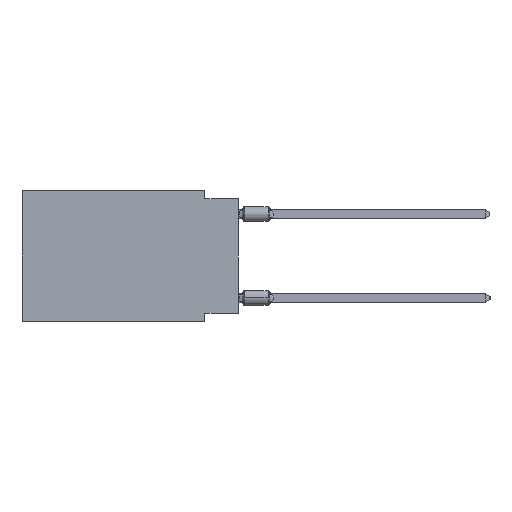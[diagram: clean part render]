
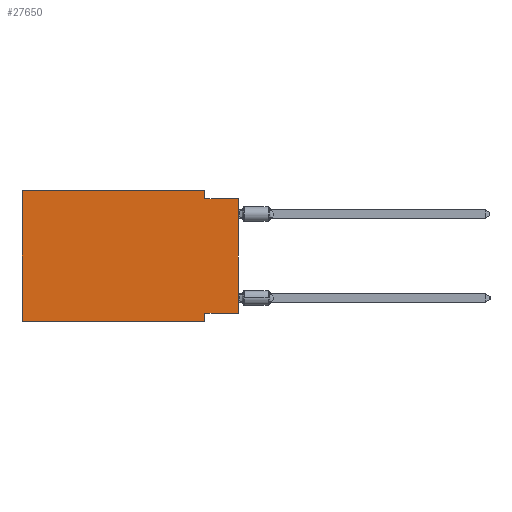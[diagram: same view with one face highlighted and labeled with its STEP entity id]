
A CAD part, left-side view. The second image highlights one B-rep face of the part: STEP entity #27650.
In plain terms, the highlighted planar face has unit normal (-1, 0, 0).
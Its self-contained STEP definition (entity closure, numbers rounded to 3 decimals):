
#1612 = EDGE_LOOP ( 'NONE', ( #21634, #5276, #21179, #56084, #26722, #26345, #9311, #29077 ) ) ;
#1823 = CARTESIAN_POINT ( 'NONE',  ( 0., 16.383, -9.906 ) ) ;
#1859 = LINE ( 'NONE', #18816, #7749 ) ;
#1873 = CARTESIAN_POINT ( 'NONE',  ( 0., 16.383, -9.906 ) ) ;
#2757 = CARTESIAN_POINT ( 'NONE',  ( 0., 16.383, 0. ) ) ;
#5276 = ORIENTED_EDGE ( 'NONE', *, *, #14238, .F. ) ;
#5579 = DIRECTION ( 'NONE',  ( 0., 0., -1. ) ) ;
#7749 = VECTOR ( 'NONE', #54801, 1000. ) ;
#7827 = VECTOR ( 'NONE', #45224, 1000. ) ;
#9311 = ORIENTED_EDGE ( 'NONE', *, *, #21600, .F. ) ;
#10253 = EDGE_CURVE ( 'NONE', #53155, #46150, #13075, .T. ) ;
#12201 = VERTEX_POINT ( 'NONE', #24061 ) ;
#12970 = LINE ( 'NONE', #40441, #18090 ) ;
#13075 = LINE ( 'NONE', #35859, #7827 ) ;
#14238 = EDGE_CURVE ( 'NONE', #12201, #20989, #27750, .T. ) ;
#15190 = EDGE_CURVE ( 'NONE', #28100, #45159, #24378, .T. ) ;
#15457 = DIRECTION ( 'NONE',  ( 0., -1., 0. ) ) ;
#18020 = VECTOR ( 'NONE', #5579, 1000. ) ;
#18090 = VECTOR ( 'NONE', #25851, 1000. ) ;
#18555 = CARTESIAN_POINT ( 'NONE',  ( 0., 16.383, 0. ) ) ;
#18816 = CARTESIAN_POINT ( 'NONE',  ( 0., 2.54, -9.906 ) ) ;
#18846 = DIRECTION ( 'NONE',  ( 0., 0., 1. ) ) ;
#19607 = AXIS2_PLACEMENT_3D ( 'NONE', #2757, #20572, #56268 ) ;
#19985 = DIRECTION ( 'NONE',  ( 0., -1., 0. ) ) ;
#20572 = DIRECTION ( 'NONE',  ( 1., 0., 0. ) ) ;
#20989 = VERTEX_POINT ( 'NONE', #35067 ) ;
#21179 = ORIENTED_EDGE ( 'NONE', *, *, #44944, .F. ) ;
#21447 = VECTOR ( 'NONE', #15457, 1000. ) ;
#21600 = EDGE_CURVE ( 'NONE', #46886, #45159, #1859, .T. ) ;
#21634 = ORIENTED_EDGE ( 'NONE', *, *, #22814, .T. ) ;
#22814 = EDGE_CURVE ( 'NONE', #47671, #20989, #12970, .T. ) ;
#24061 = CARTESIAN_POINT ( 'NONE',  ( 0., 2.54, -0.635 ) ) ;
#24378 = LINE ( 'NONE', #1873, #30721 ) ;
#24969 = FACE_OUTER_BOUND ( 'NONE', #1612, .T. ) ;
#25851 = DIRECTION ( 'NONE',  ( 0., 0., 1. ) ) ;
#26101 = EDGE_CURVE ( 'NONE', #47671, #46886, #44420, .T. ) ;
#26306 = CARTESIAN_POINT ( 'NONE',  ( 0., 0., -9.271 ) ) ;
#26345 = ORIENTED_EDGE ( 'NONE', *, *, #15190, .T. ) ;
#26722 = ORIENTED_EDGE ( 'NONE', *, *, #49243, .F. ) ;
#27650 = ADVANCED_FACE ( 'NONE', ( #24969 ), #29928, .F. ) ;
#27750 = LINE ( 'NONE', #54671, #21447 ) ;
#28100 = VERTEX_POINT ( 'NONE', #1823 ) ;
#29077 = ORIENTED_EDGE ( 'NONE', *, *, #26101, .F. ) ;
#29928 = PLANE ( 'NONE',  #19607 ) ;
#30409 = CARTESIAN_POINT ( 'NONE',  ( 0., 2.54, -9.906 ) ) ;
#30721 = VECTOR ( 'NONE', #19985, 1000. ) ;
#32488 = CARTESIAN_POINT ( 'NONE',  ( 0., 2.54, 0. ) ) ;
#33449 = VECTOR ( 'NONE', #44133, 1000. ) ;
#34519 = CARTESIAN_POINT ( 'NONE',  ( 0., 2.54, -9.271 ) ) ;
#35067 = CARTESIAN_POINT ( 'NONE',  ( 0., 0., -0.635 ) ) ;
#35859 = CARTESIAN_POINT ( 'NONE',  ( 0., 16.383, 0. ) ) ;
#40441 = CARTESIAN_POINT ( 'NONE',  ( 0., 0., 0. ) ) ;
#44133 = DIRECTION ( 'NONE',  ( 0., 1., 0. ) ) ;
#44420 = LINE ( 'NONE', #26306, #33449 ) ;
#44877 = LINE ( 'NONE', #18555, #54701 ) ;
#44944 = EDGE_CURVE ( 'NONE', #46150, #12201, #50614, .T. ) ;
#45159 = VERTEX_POINT ( 'NONE', #30409 ) ;
#45224 = DIRECTION ( 'NONE',  ( 0., -1., 0. ) ) ;
#46150 = VERTEX_POINT ( 'NONE', #46527 ) ;
#46527 = CARTESIAN_POINT ( 'NONE',  ( 0., 2.54, 0. ) ) ;
#46886 = VERTEX_POINT ( 'NONE', #34519 ) ;
#47671 = VERTEX_POINT ( 'NONE', #53737 ) ;
#49243 = EDGE_CURVE ( 'NONE', #28100, #53155, #44877, .T. ) ;
#50614 = LINE ( 'NONE', #32488, #18020 ) ;
#53155 = VERTEX_POINT ( 'NONE', #57645 ) ;
#53737 = CARTESIAN_POINT ( 'NONE',  ( 0., 0., -9.271 ) ) ;
#54671 = CARTESIAN_POINT ( 'NONE',  ( 0., 0., -0.635 ) ) ;
#54701 = VECTOR ( 'NONE', #18846, 1000. ) ;
#54801 = DIRECTION ( 'NONE',  ( 0., 0., -1. ) ) ;
#56084 = ORIENTED_EDGE ( 'NONE', *, *, #10253, .F. ) ;
#56268 = DIRECTION ( 'NONE',  ( 0., 0., -1. ) ) ;
#57645 = CARTESIAN_POINT ( 'NONE',  ( 0., 16.383, 0. ) ) ;
